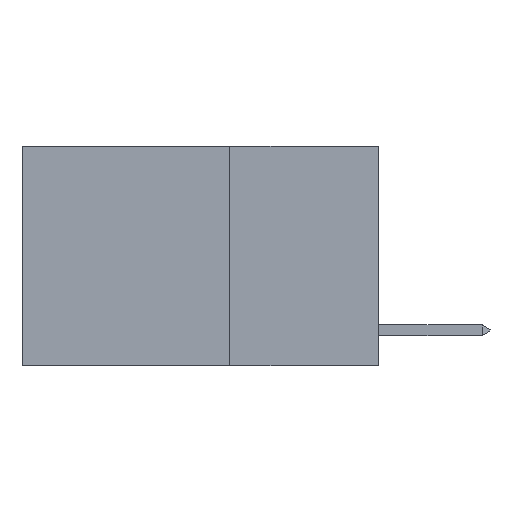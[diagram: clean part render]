
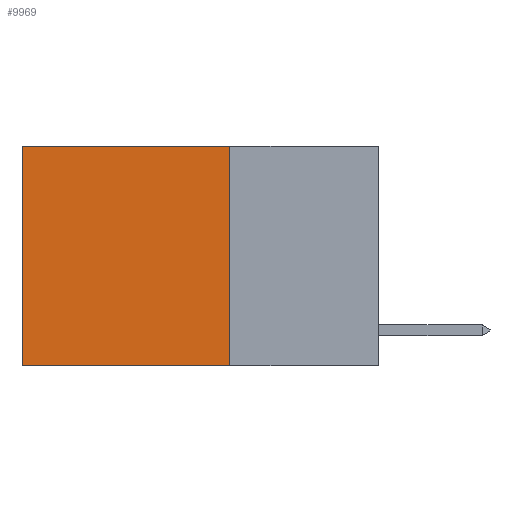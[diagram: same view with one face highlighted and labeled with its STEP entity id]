
A CAD part, left-side view. The second image highlights one B-rep face of the part: STEP entity #9969.
In plain terms, the highlighted planar face has unit normal (-1, 0, 0).
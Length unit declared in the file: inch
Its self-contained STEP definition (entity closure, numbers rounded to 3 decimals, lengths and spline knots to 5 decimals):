
#191 = ORIENTED_EDGE ( 'NONE', *, *, #1275, .T. ) ;
#1061 = EDGE_LOOP ( 'NONE', ( #1883, #4367, #9410, #191 ) ) ;
#1064 = EDGE_CURVE ( 'NONE', #9135, #2472, #12242, .T. ) ;
#1275 = EDGE_CURVE ( 'NONE', #9135, #2527, #10556, .T. ) ;
#1788 = CARTESIAN_POINT ( 'NONE',  ( 0.2625, 0.25, -0.37 ) ) ;
#1883 = ORIENTED_EDGE ( 'NONE', *, *, #5121, .T. ) ;
#2150 = CARTESIAN_POINT ( 'NONE',  ( 0.2625, 0.25, 0. ) ) ;
#2472 = VERTEX_POINT ( 'NONE', #1788 ) ;
#2527 = VERTEX_POINT ( 'NONE', #10498 ) ;
#3831 = DIRECTION ( 'NONE',  ( 0., 1., 0. ) ) ;
#3892 = PLANE ( 'NONE',  #6694 ) ;
#4367 = ORIENTED_EDGE ( 'NONE', *, *, #8363, .F. ) ;
#4382 = LINE ( 'NONE', #8674, #6152 ) ;
#4862 = DIRECTION ( 'NONE',  ( 1., 0., 0. ) ) ;
#5121 = EDGE_CURVE ( 'NONE', #2527, #6304, #10690, .T. ) ;
#5388 = FACE_OUTER_BOUND ( 'NONE', #1061, .T. ) ;
#5713 = CARTESIAN_POINT ( 'NONE',  ( 0.2625, 0.25, 0. ) ) ;
#6152 = VECTOR ( 'NONE', #3831, 39.37008 ) ;
#6304 = VERTEX_POINT ( 'NONE', #12487 ) ;
#6694 = AXIS2_PLACEMENT_3D ( 'NONE', #9645, #4862, #8607 ) ;
#7740 = DIRECTION ( 'NONE',  ( 0., 0., -1. ) ) ;
#7976 = VECTOR ( 'NONE', #10713, 39.37008 ) ;
#8363 = EDGE_CURVE ( 'NONE', #2472, #6304, #4382, .T. ) ;
#8607 = DIRECTION ( 'NONE',  ( 0., 0., -1. ) ) ;
#8674 = CARTESIAN_POINT ( 'NONE',  ( 0.2625, 0.25, -0.37 ) ) ;
#9135 = VERTEX_POINT ( 'NONE', #10149 ) ;
#9410 = ORIENTED_EDGE ( 'NONE', *, *, #1064, .F. ) ;
#9645 = CARTESIAN_POINT ( 'NONE',  ( 0.2625, 0.25, 0. ) ) ;
#9969 = ADVANCED_FACE ( 'NONE', ( #5388 ), #3892, .F. ) ;
#10035 = DIRECTION ( 'NONE',  ( 0., 1., 0. ) ) ;
#10149 = CARTESIAN_POINT ( 'NONE',  ( 0.2625, 0.25, 0. ) ) ;
#10498 = CARTESIAN_POINT ( 'NONE',  ( 0.2625, 0.6, 0. ) ) ;
#10556 = LINE ( 'NONE', #2150, #12539 ) ;
#10588 = CARTESIAN_POINT ( 'NONE',  ( 0.2625, 0.6, 0. ) ) ;
#10690 = LINE ( 'NONE', #10588, #7976 ) ;
#10713 = DIRECTION ( 'NONE',  ( 0., 0., -1. ) ) ;
#12090 = VECTOR ( 'NONE', #7740, 39.37008 ) ;
#12242 = LINE ( 'NONE', #5713, #12090 ) ;
#12487 = CARTESIAN_POINT ( 'NONE',  ( 0.2625, 0.6, -0.37 ) ) ;
#12539 = VECTOR ( 'NONE', #10035, 39.37008 ) ;
